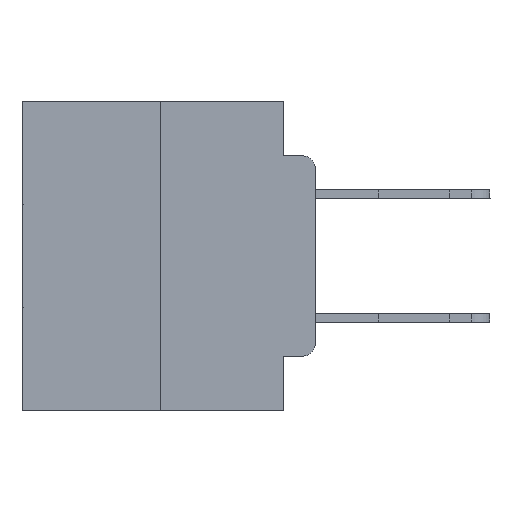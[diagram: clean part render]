
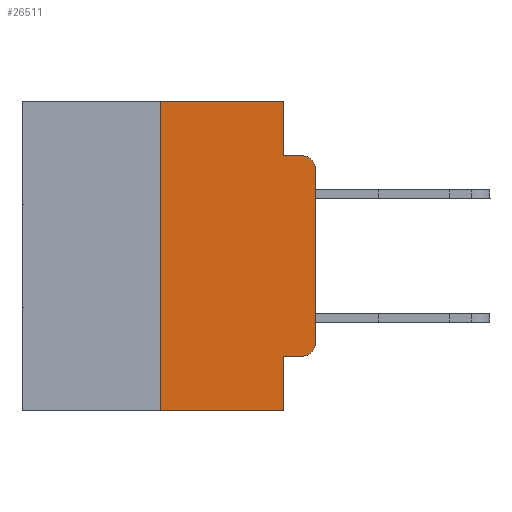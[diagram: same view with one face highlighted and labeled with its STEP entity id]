
A CAD part, left-side view. The second image highlights one B-rep face of the part: STEP entity #26511.
In plain terms, the highlighted planar face has unit normal (-1, 0, 0).
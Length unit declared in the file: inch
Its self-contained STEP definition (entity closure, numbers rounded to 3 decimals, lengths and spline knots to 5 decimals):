
#170 = EDGE_CURVE ( 'NONE', #9093, #28533, #26202, .T. ) ;
#757 = CARTESIAN_POINT ( 'NONE',  ( 0., 0.473, 0. ) ) ;
#862 = CARTESIAN_POINT ( 'NONE',  ( 0., 0.02, -0.3915 ) ) ;
#1901 = EDGE_CURVE ( 'NONE', #28533, #7713, #25399, .T. ) ;
#2192 = LINE ( 'NONE', #9607, #8746 ) ;
#2790 = DIRECTION ( 'NONE',  ( 0., 0., -1. ) ) ;
#3110 = VECTOR ( 'NONE', #24559, 39.37008 ) ;
#3155 = ORIENTED_EDGE ( 'NONE', *, *, #1901, .T. ) ;
#3537 = CARTESIAN_POINT ( 'NONE',  ( 0., 0.02, -0.0885 ) ) ;
#3644 = ORIENTED_EDGE ( 'NONE', *, *, #24995, .F. ) ;
#3664 = CARTESIAN_POINT ( 'NONE',  ( 0., 0.051, -0.0885 ) ) ;
#4153 = CARTESIAN_POINT ( 'NONE',  ( 0., 0.25, 0. ) ) ;
#4498 = ORIENTED_EDGE ( 'NONE', *, *, #170, .T. ) ;
#4904 = CARTESIAN_POINT ( 'NONE',  ( 0., 0.473, -0.5 ) ) ;
#5037 = CARTESIAN_POINT ( 'NONE',  ( 0., 0.051, -0.5 ) ) ;
#5261 = DIRECTION ( 'NONE',  ( 0., 0., -1. ) ) ;
#5486 = CARTESIAN_POINT ( 'NONE',  ( 0., 0.02, -0.4115 ) ) ;
#5605 = EDGE_CURVE ( 'NONE', #16660, #24719, #26085, .T. ) ;
#5677 = VECTOR ( 'NONE', #24524, 39.37008 ) ;
#7479 = AXIS2_PLACEMENT_3D ( 'NONE', #20850, #22942, #5261 ) ;
#7713 = VERTEX_POINT ( 'NONE', #3537 ) ;
#7840 = VERTEX_POINT ( 'NONE', #21467 ) ;
#8523 = LINE ( 'NONE', #28263, #24026 ) ;
#8717 = CARTESIAN_POINT ( 'NONE',  ( 0., 0.051, -0.4115 ) ) ;
#8746 = VECTOR ( 'NONE', #14151, 39.37008 ) ;
#9009 = EDGE_CURVE ( 'NONE', #10897, #17682, #17964, .T. ) ;
#9093 = VERTEX_POINT ( 'NONE', #15234 ) ;
#9549 = VECTOR ( 'NONE', #16727, 39.37008 ) ;
#9607 = CARTESIAN_POINT ( 'NONE',  ( 0., 0.25, 0. ) ) ;
#10323 = DIRECTION ( 'NONE',  ( 0., 0., -1. ) ) ;
#10897 = VERTEX_POINT ( 'NONE', #8717 ) ;
#10932 = CARTESIAN_POINT ( 'NONE',  ( 0., 0.051, 0. ) ) ;
#11273 = CIRCLE ( 'NONE', #18141, 0.02 ) ;
#11377 = AXIS2_PLACEMENT_3D ( 'NONE', #757, #19084, #10323 ) ;
#11675 = PLANE ( 'NONE',  #11377 ) ;
#12566 = CARTESIAN_POINT ( 'NONE',  ( 0., 0.473, 0. ) ) ;
#12926 = VECTOR ( 'NONE', #24997, 39.37008 ) ;
#14151 = DIRECTION ( 'NONE',  ( 0., 0., 1. ) ) ;
#14936 = ORIENTED_EDGE ( 'NONE', *, *, #5605, .F. ) ;
#15234 = CARTESIAN_POINT ( 'NONE',  ( 0., 0., -0.3915 ) ) ;
#15790 = ORIENTED_EDGE ( 'NONE', *, *, #28272, .T. ) ;
#15886 = EDGE_LOOP ( 'NONE', ( #4498, #3155, #22820, #14936, #3644, #17745, #15953, #27926, #15790, #22779 ) ) ;
#15953 = ORIENTED_EDGE ( 'NONE', *, *, #24949, .T. ) ;
#16466 = LINE ( 'NONE', #12566, #9549 ) ;
#16660 = VERTEX_POINT ( 'NONE', #19051 ) ;
#16727 = DIRECTION ( 'NONE',  ( 0., -1., 0. ) ) ;
#17309 = VECTOR ( 'NONE', #21726, 39.37008 ) ;
#17682 = VERTEX_POINT ( 'NONE', #5037 ) ;
#17745 = ORIENTED_EDGE ( 'NONE', *, *, #19503, .F. ) ;
#17757 = EDGE_CURVE ( 'NONE', #21388, #9093, #11273, .T. ) ;
#17964 = LINE ( 'NONE', #10932, #17309 ) ;
#18141 = AXIS2_PLACEMENT_3D ( 'NONE', #862, #18614, #25332 ) ;
#18303 = FACE_OUTER_BOUND ( 'NONE', #15886, .T. ) ;
#18523 = VERTEX_POINT ( 'NONE', #4153 ) ;
#18614 = DIRECTION ( 'NONE',  ( -1., 0., 0. ) ) ;
#19051 = CARTESIAN_POINT ( 'NONE',  ( 0., 0.051, 0. ) ) ;
#19084 = DIRECTION ( 'NONE',  ( 1., 0., 0. ) ) ;
#19459 = LINE ( 'NONE', #22769, #12926 ) ;
#19503 = EDGE_CURVE ( 'NONE', #7840, #18523, #2192, .T. ) ;
#20850 = CARTESIAN_POINT ( 'NONE',  ( 0., 0.02, -0.1085 ) ) ;
#21388 = VERTEX_POINT ( 'NONE', #5486 ) ;
#21467 = CARTESIAN_POINT ( 'NONE',  ( 0., 0.25, -0.5 ) ) ;
#21726 = DIRECTION ( 'NONE',  ( 0., 0., -1. ) ) ;
#22769 = CARTESIAN_POINT ( 'NONE',  ( 0., 0.051, -0.0885 ) ) ;
#22779 = ORIENTED_EDGE ( 'NONE', *, *, #17757, .T. ) ;
#22820 = ORIENTED_EDGE ( 'NONE', *, *, #23107, .F. ) ;
#22859 = LINE ( 'NONE', #4904, #5677 ) ;
#22942 = DIRECTION ( 'NONE',  ( -1., 0., 0. ) ) ;
#23107 = EDGE_CURVE ( 'NONE', #24719, #7713, #19459, .T. ) ;
#24026 = VECTOR ( 'NONE', #27892, 39.37008 ) ;
#24357 = VECTOR ( 'NONE', #2790, 39.37008 ) ;
#24524 = DIRECTION ( 'NONE',  ( 0., -1., 0. ) ) ;
#24559 = DIRECTION ( 'NONE',  ( 0., 0., 1. ) ) ;
#24719 = VERTEX_POINT ( 'NONE', #3664 ) ;
#24949 = EDGE_CURVE ( 'NONE', #7840, #17682, #22859, .T. ) ;
#24995 = EDGE_CURVE ( 'NONE', #18523, #16660, #16466, .T. ) ;
#24997 = DIRECTION ( 'NONE',  ( 0., -1., 0. ) ) ;
#25332 = DIRECTION ( 'NONE',  ( 0., 0., -1. ) ) ;
#25341 = CARTESIAN_POINT ( 'NONE',  ( 0., 0.051, 0. ) ) ;
#25399 = CIRCLE ( 'NONE', #7479, 0.02 ) ;
#26085 = LINE ( 'NONE', #25341, #24357 ) ;
#26202 = LINE ( 'NONE', #26871, #3110 ) ;
#26511 = ADVANCED_FACE ( 'NONE', ( #18303 ), #11675, .F. ) ;
#26871 = CARTESIAN_POINT ( 'NONE',  ( 0., 0., 0. ) ) ;
#27560 = CARTESIAN_POINT ( 'NONE',  ( 0., 0., -0.1085 ) ) ;
#27892 = DIRECTION ( 'NONE',  ( 0., -1., 0. ) ) ;
#27926 = ORIENTED_EDGE ( 'NONE', *, *, #9009, .F. ) ;
#28263 = CARTESIAN_POINT ( 'NONE',  ( 0., 0.051, -0.4115 ) ) ;
#28272 = EDGE_CURVE ( 'NONE', #10897, #21388, #8523, .T. ) ;
#28533 = VERTEX_POINT ( 'NONE', #27560 ) ;
